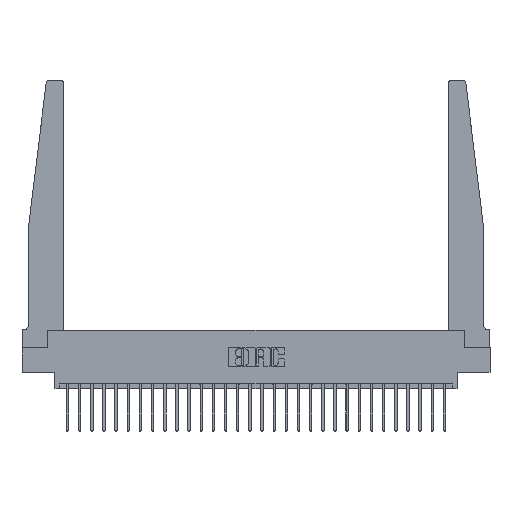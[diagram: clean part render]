
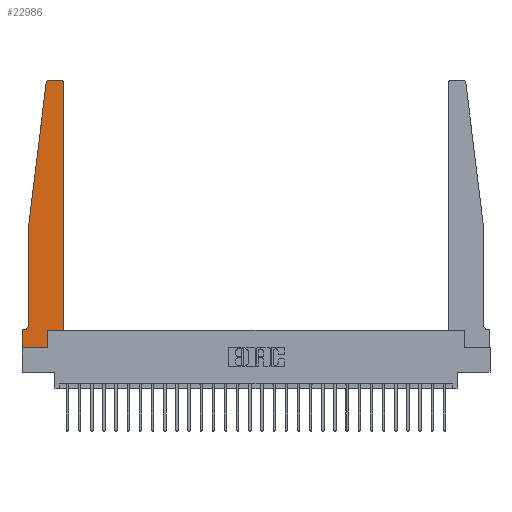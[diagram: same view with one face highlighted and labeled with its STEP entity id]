
A CAD part, top view. The second image highlights one B-rep face of the part: STEP entity #22986.
In plain terms, the highlighted planar face has unit normal (0, 0, 1).
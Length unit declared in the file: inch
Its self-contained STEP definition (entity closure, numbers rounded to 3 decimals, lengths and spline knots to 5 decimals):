
#956 = CARTESIAN_POINT ( 'NONE',  ( 0.065, 1.25, 0.37 ) ) ;
#1008 = VERTEX_POINT ( 'NONE', #21663 ) ;
#1182 = ORIENTED_EDGE ( 'NONE', *, *, #16230, .T. ) ;
#1521 = CIRCLE ( 'NONE', #2911, 0.05 ) ;
#2038 = DIRECTION ( 'NONE',  ( 0., 1., 0. ) ) ;
#2072 = FACE_OUTER_BOUND ( 'NONE', #27572, .T. ) ;
#2175 = ORIENTED_EDGE ( 'NONE', *, *, #9251, .T. ) ;
#2408 = ORIENTED_EDGE ( 'NONE', *, *, #23046, .T. ) ;
#2910 = VECTOR ( 'NONE', #25848, 39.37008 ) ;
#2911 = AXIS2_PLACEMENT_3D ( 'NONE', #12183, #18598, #24617 ) ;
#3525 = EDGE_CURVE ( 'NONE', #26314, #23877, #1521, .T. ) ;
#3737 = LINE ( 'NONE', #5726, #25591 ) ;
#3774 = CIRCLE ( 'NONE', #19434, 0.03 ) ;
#3908 = CARTESIAN_POINT ( 'NONE',  ( 0.395, 2.75, 0.37 ) ) ;
#4866 = DIRECTION ( 'NONE',  ( 0., 0., 1. ) ) ;
#4874 = LINE ( 'NONE', #17330, #25943 ) ;
#5541 = VECTOR ( 'NONE', #11625, 39.37008 ) ;
#5627 = VERTEX_POINT ( 'NONE', #6774 ) ;
#5726 = CARTESIAN_POINT ( 'NONE',  ( 0.425, 0.18, 0.37 ) ) ;
#6088 = ORIENTED_EDGE ( 'NONE', *, *, #9028, .T. ) ;
#6376 = ORIENTED_EDGE ( 'NONE', *, *, #9639, .T. ) ;
#6539 = CARTESIAN_POINT ( 'NONE',  ( 0., 0., 0.37 ) ) ;
#6774 = CARTESIAN_POINT ( 'NONE',  ( 0.24675, 2.72367, 0.37 ) ) ;
#8191 = CARTESIAN_POINT ( 'NONE',  ( 0.395, 2.72, 0.37 ) ) ;
#8504 = LINE ( 'NONE', #17004, #24318 ) ;
#9028 = EDGE_CURVE ( 'NONE', #1008, #26437, #22200, .T. ) ;
#9251 = EDGE_CURVE ( 'NONE', #22937, #24401, #8504, .T. ) ;
#9266 = CARTESIAN_POINT ( 'NONE',  ( 0.065, 0.1875, 0.37 ) ) ;
#9639 = EDGE_CURVE ( 'NONE', #12483, #22937, #3774, .T. ) ;
#9644 = CARTESIAN_POINT ( 'NONE',  ( 0.065, 0.2375, 0.37 ) ) ;
#10391 = CARTESIAN_POINT ( 'NONE',  ( 0.425, 2.72, 0.37 ) ) ;
#11068 = DIRECTION ( 'NONE',  ( 1., 0., 0. ) ) ;
#11152 = DIRECTION ( 'NONE',  ( -1., 0., 0. ) ) ;
#11473 = CARTESIAN_POINT ( 'NONE',  ( 0., 0., 0.37 ) ) ;
#11625 = DIRECTION ( 'NONE',  ( -0.122, -0.992, 0. ) ) ;
#12010 = CARTESIAN_POINT ( 'NONE',  ( 0.2605, 0., 0.37 ) ) ;
#12120 = DIRECTION ( 'NONE',  ( 1., 0., 0. ) ) ;
#12169 = DIRECTION ( 'NONE',  ( 0., 1., 0. ) ) ;
#12183 = CARTESIAN_POINT ( 'NONE',  ( 0.015, 0.2375, 0.37 ) ) ;
#12483 = VERTEX_POINT ( 'NONE', #10391 ) ;
#12687 = CARTESIAN_POINT ( 'NONE',  ( 0., 0., 0.37 ) ) ;
#12898 = CARTESIAN_POINT ( 'NONE',  ( 0.065, 1.25, 0.37 ) ) ;
#13706 = DIRECTION ( 'NONE',  ( 1., 0., 0. ) ) ;
#13979 = DIRECTION ( 'NONE',  ( 0., -1., 0. ) ) ;
#14147 = ORIENTED_EDGE ( 'NONE', *, *, #23158, .T. ) ;
#14402 = EDGE_CURVE ( 'NONE', #27336, #24684, #18705, .T. ) ;
#14484 = CIRCLE ( 'NONE', #18921, 0.03 ) ;
#14943 = VECTOR ( 'NONE', #20341, 39.37008 ) ;
#16230 = EDGE_CURVE ( 'NONE', #26437, #27336, #27295, .T. ) ;
#16541 = CARTESIAN_POINT ( 'NONE',  ( 0.425, 0.18, 0.37 ) ) ;
#16695 = DIRECTION ( 'NONE',  ( 0., 0., 1. ) ) ;
#17004 = CARTESIAN_POINT ( 'NONE',  ( 0.25, 2.75, 0.37 ) ) ;
#17174 = VECTOR ( 'NONE', #13979, 39.37008 ) ;
#17214 = CARTESIAN_POINT ( 'NONE',  ( 0., 0.1875, 0.37 ) ) ;
#17330 = CARTESIAN_POINT ( 'NONE',  ( 0.065, 1.25, 0.37 ) ) ;
#17549 = EDGE_CURVE ( 'NONE', #21911, #26314, #4874, .T. ) ;
#18470 = VECTOR ( 'NONE', #2038, 39.37008 ) ;
#18598 = DIRECTION ( 'NONE',  ( 0., 0., -1. ) ) ;
#18705 = LINE ( 'NONE', #24989, #18470 ) ;
#18795 = ORIENTED_EDGE ( 'NONE', *, *, #26618, .T. ) ;
#18921 = AXIS2_PLACEMENT_3D ( 'NONE', #24010, #4866, #13706 ) ;
#19434 = AXIS2_PLACEMENT_3D ( 'NONE', #8191, #16695, #12120 ) ;
#19834 = CARTESIAN_POINT ( 'NONE',  ( 0.425, 0.18, 0.37 ) ) ;
#20145 = CARTESIAN_POINT ( 'NONE',  ( 0.27653, 2.75, 0.37 ) ) ;
#20341 = DIRECTION ( 'NONE',  ( 1., 0., 0. ) ) ;
#21065 = ORIENTED_EDGE ( 'NONE', *, *, #14402, .T. ) ;
#21382 = LINE ( 'NONE', #9266, #2910 ) ;
#21663 = CARTESIAN_POINT ( 'NONE',  ( 0., 0.1875, 0.37 ) ) ;
#21909 = ORIENTED_EDGE ( 'NONE', *, *, #26020, .T. ) ;
#21911 = VERTEX_POINT ( 'NONE', #12898 ) ;
#21931 = ORIENTED_EDGE ( 'NONE', *, *, #3525, .T. ) ;
#22200 = LINE ( 'NONE', #11473, #17174 ) ;
#22654 = ORIENTED_EDGE ( 'NONE', *, *, #27281, .T. ) ;
#22937 = VERTEX_POINT ( 'NONE', #3908 ) ;
#22986 = ADVANCED_FACE ( 'NONE', ( #2072 ), #25434, .T. ) ;
#22992 = CARTESIAN_POINT ( 'NONE',  ( 0.015, 0.1875, 0.37 ) ) ;
#23046 = EDGE_CURVE ( 'NONE', #5627, #21911, #26267, .T. ) ;
#23158 = EDGE_CURVE ( 'NONE', #26143, #12483, #3737, .T. ) ;
#23595 = CARTESIAN_POINT ( 'NONE',  ( 0.2605, 0.18, 0.37 ) ) ;
#23877 = VERTEX_POINT ( 'NONE', #22992 ) ;
#24010 = CARTESIAN_POINT ( 'NONE',  ( 0.27653, 2.72, 0.37 ) ) ;
#24046 = DIRECTION ( 'NONE',  ( 0., 0., 1. ) ) ;
#24271 = AXIS2_PLACEMENT_3D ( 'NONE', #17214, #24046, #11068 ) ;
#24318 = VECTOR ( 'NONE', #11152, 39.37008 ) ;
#24401 = VERTEX_POINT ( 'NONE', #20145 ) ;
#24617 = DIRECTION ( 'NONE',  ( -1., 0., 0. ) ) ;
#24684 = VERTEX_POINT ( 'NONE', #23595 ) ;
#24695 = ORIENTED_EDGE ( 'NONE', *, *, #17549, .T. ) ;
#24989 = CARTESIAN_POINT ( 'NONE',  ( 0.2605, 0.18, 0.37 ) ) ;
#25434 = PLANE ( 'NONE',  #24271 ) ;
#25439 = VECTOR ( 'NONE', #25919, 39.37008 ) ;
#25591 = VECTOR ( 'NONE', #12169, 39.37008 ) ;
#25821 = DIRECTION ( 'NONE',  ( 0., -1., 0. ) ) ;
#25848 = DIRECTION ( 'NONE',  ( -1., 0., 0. ) ) ;
#25919 = DIRECTION ( 'NONE',  ( 1., 0., 0. ) ) ;
#25943 = VECTOR ( 'NONE', #25821, 39.37008 ) ;
#26020 = EDGE_CURVE ( 'NONE', #24401, #5627, #14484, .T. ) ;
#26143 = VERTEX_POINT ( 'NONE', #19834 ) ;
#26267 = LINE ( 'NONE', #956, #5541 ) ;
#26314 = VERTEX_POINT ( 'NONE', #9644 ) ;
#26437 = VERTEX_POINT ( 'NONE', #12687 ) ;
#26618 = EDGE_CURVE ( 'NONE', #24684, #26143, #26736, .T. ) ;
#26736 = LINE ( 'NONE', #16541, #14943 ) ;
#27281 = EDGE_CURVE ( 'NONE', #23877, #1008, #21382, .T. ) ;
#27295 = LINE ( 'NONE', #6539, #25439 ) ;
#27336 = VERTEX_POINT ( 'NONE', #12010 ) ;
#27572 = EDGE_LOOP ( 'NONE', ( #2175, #21909, #2408, #24695, #21931, #22654, #6088, #1182, #21065, #18795, #14147, #6376 ) ) ;
